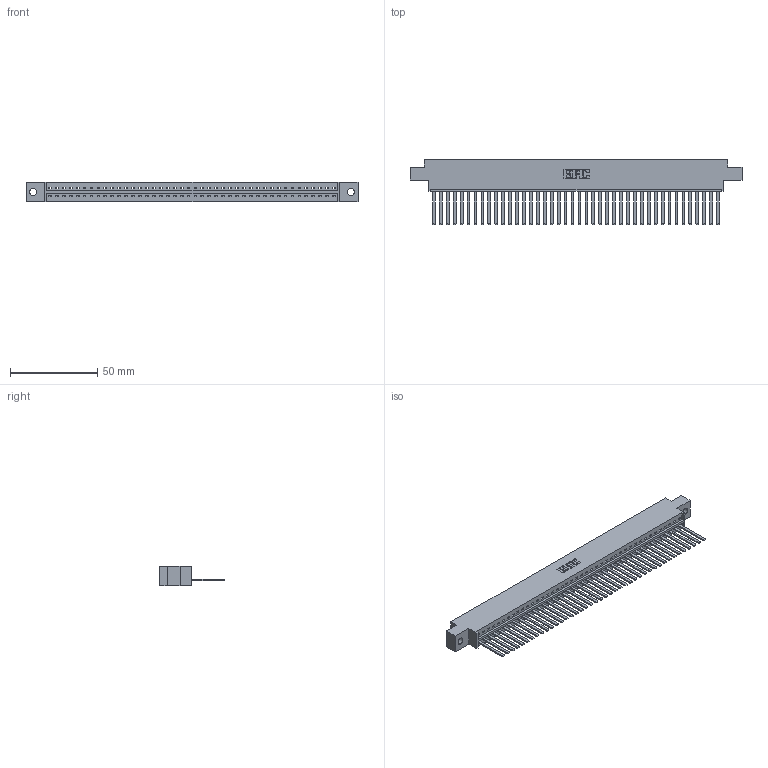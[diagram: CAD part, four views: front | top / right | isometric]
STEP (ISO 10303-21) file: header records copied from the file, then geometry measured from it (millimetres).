
FILE_DESCRIPTION (( 'STEP AP203' ), '1' );
FILE_NAME ('336-042-541-604.STEP', '2020-08-07T23:33:59', ( '' ), ( '' ), 'SwSTEP 2.0', 'SolidWorks 2020', '' );
FILE_SCHEMA (( 'CONFIG_CONTROL_DESIGN' ));
Length unit declared in the file: inch
Products named in the file (3): 336 Part_Offset - .156 Dia - TH; 336-290-001_336-290-541; 336-042-541-604
Assembly tree (43 placements, depth 2):
  336-042-541-604
    336 Part_Offset - .156 Dia - TH
    336-290-001_336-290-541  x42
Bounding box: 189.81 x 37.34 x 11.1 mm (x, y, z)
Volume: 27567.9 mm3; surface area: 29886.8 mm2
Topology: 43 solids, 43 shells, 2218 faces, 6791 edges, 4498 vertices
Faces by surface type: plane 1502, cylinder 716
Entity records: 31074 total; most frequent: CARTESIAN_POINT 5503, ORIENTED_EDGE 5382, DIRECTION 4535, EDGE_CURVE 2691, VECTOR 2559, LINE 2559, VERTEX_POINT 1792, AXIS2_PLACEMENT_3D 988
